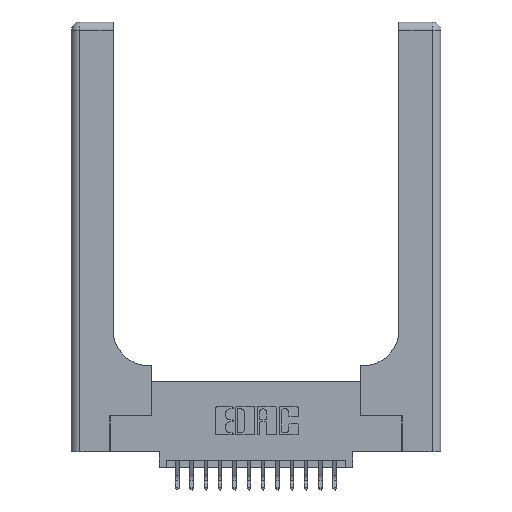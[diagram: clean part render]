
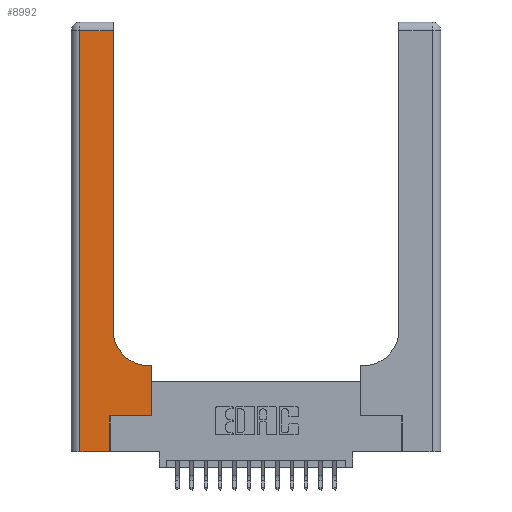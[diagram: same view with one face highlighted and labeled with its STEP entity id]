
A CAD part, top view. The second image highlights one B-rep face of the part: STEP entity #8992.
In plain terms, the highlighted planar face has unit normal (0, 0, 1).
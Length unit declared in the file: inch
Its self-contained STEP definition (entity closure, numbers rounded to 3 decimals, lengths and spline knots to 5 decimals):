
#771 = ORIENTED_EDGE ( 'NONE', *, *, #18063, .T. ) ;
#1486 = VECTOR ( 'NONE', #8762, 39.37008 ) ;
#1741 = CARTESIAN_POINT ( 'NONE',  ( 0.2915, 2.94, 0.37 ) ) ;
#1759 = VERTEX_POINT ( 'NONE', #3082 ) ;
#1882 = EDGE_CURVE ( 'NONE', #12245, #2724, #18890, .T. ) ;
#1940 = DIRECTION ( 'NONE',  ( 0., 1., 0. ) ) ;
#2143 = CARTESIAN_POINT ( 'NONE',  ( 0.269, 0., 0.37 ) ) ;
#2274 = VECTOR ( 'NONE', #14615, 39.37008 ) ;
#2296 = CARTESIAN_POINT ( 'NONE',  ( 0.5415, 0.6, 0.37 ) ) ;
#2349 = CARTESIAN_POINT ( 'NONE',  ( 0., 2.94, 0.37 ) ) ;
#2434 = ORIENTED_EDGE ( 'NONE', *, *, #6491, .T. ) ;
#2440 = VERTEX_POINT ( 'NONE', #1741 ) ;
#2676 = LINE ( 'NONE', #6686, #13928 ) ;
#2724 = VERTEX_POINT ( 'NONE', #4999 ) ;
#3082 = CARTESIAN_POINT ( 'NONE',  ( 0.5585, 0.25, 0.37 ) ) ;
#3432 = CARTESIAN_POINT ( 'NONE',  ( 0.269, 0.25, 0.37 ) ) ;
#3605 = ORIENTED_EDGE ( 'NONE', *, *, #11984, .T. ) ;
#3850 = LINE ( 'NONE', #18916, #2274 ) ;
#4032 = DIRECTION ( 'NONE',  ( 0., -1., 0. ) ) ;
#4252 = LINE ( 'NONE', #7621, #5389 ) ;
#4438 = VECTOR ( 'NONE', #16854, 39.37008 ) ;
#4523 = VERTEX_POINT ( 'NONE', #18541 ) ;
#4768 = ORIENTED_EDGE ( 'NONE', *, *, #18151, .T. ) ;
#4783 = VERTEX_POINT ( 'NONE', #13072 ) ;
#4784 = CARTESIAN_POINT ( 'NONE',  ( 0., 0., 0.37 ) ) ;
#4999 = CARTESIAN_POINT ( 'NONE',  ( 0.2915, 0.85, 0.37 ) ) ;
#5149 = VECTOR ( 'NONE', #12621, 39.37008 ) ;
#5171 = DIRECTION ( 'NONE',  ( -1., 0., 0. ) ) ;
#5389 = VECTOR ( 'NONE', #1940, 39.37008 ) ;
#5469 = ORIENTED_EDGE ( 'NONE', *, *, #11515, .T. ) ;
#5716 = EDGE_LOOP ( 'NONE', ( #2434, #6113, #771, #4768, #14386, #7467, #5469, #3605, #16945 ) ) ;
#6108 = CARTESIAN_POINT ( 'NONE',  ( 0.5585, 0.6, 0.37 ) ) ;
#6113 = ORIENTED_EDGE ( 'NONE', *, *, #17376, .T. ) ;
#6252 = VECTOR ( 'NONE', #13471, 39.37008 ) ;
#6491 = EDGE_CURVE ( 'NONE', #2724, #2440, #2676, .T. ) ;
#6592 = DIRECTION ( 'NONE',  ( 0., 0., -1. ) ) ;
#6686 = CARTESIAN_POINT ( 'NONE',  ( 0.2915, 3., 0.37 ) ) ;
#7422 = VECTOR ( 'NONE', #4032, 39.37008 ) ;
#7467 = ORIENTED_EDGE ( 'NONE', *, *, #16045, .T. ) ;
#7542 = VERTEX_POINT ( 'NONE', #3432 ) ;
#7621 = CARTESIAN_POINT ( 'NONE',  ( 0.5585, 0.25, 0.37 ) ) ;
#8762 = DIRECTION ( 'NONE',  ( -1., 0., 0. ) ) ;
#8992 = ADVANCED_FACE ( 'NONE', ( #16774 ), #12538, .F. ) ;
#9078 = LINE ( 'NONE', #2349, #5149 ) ;
#9224 = CARTESIAN_POINT ( 'NONE',  ( 0.06, 2.94, 0.37 ) ) ;
#9923 = CARTESIAN_POINT ( 'NONE',  ( 0.06, 3., 0.37 ) ) ;
#10293 = CARTESIAN_POINT ( 'NONE',  ( 0.2915, 0.6, 0.37 ) ) ;
#11515 = EDGE_CURVE ( 'NONE', #1759, #11994, #4252, .T. ) ;
#11984 = EDGE_CURVE ( 'NONE', #11994, #12245, #13197, .T. ) ;
#11994 = VERTEX_POINT ( 'NONE', #6108 ) ;
#12245 = VERTEX_POINT ( 'NONE', #2296 ) ;
#12308 = CARTESIAN_POINT ( 'NONE',  ( 0.5415, 0.85, 0.37 ) ) ;
#12538 = PLANE ( 'NONE',  #17915 ) ;
#12621 = DIRECTION ( 'NONE',  ( -1., 0., 0. ) ) ;
#12978 = LINE ( 'NONE', #2143, #4438 ) ;
#13072 = CARTESIAN_POINT ( 'NONE',  ( 0.269, 0., 0.37 ) ) ;
#13197 = LINE ( 'NONE', #10293, #1486 ) ;
#13234 = VERTEX_POINT ( 'NONE', #9224 ) ;
#13471 = DIRECTION ( 'NONE',  ( 1., 0., 0. ) ) ;
#13798 = DIRECTION ( 'NONE',  ( 0., 0., -1. ) ) ;
#13928 = VECTOR ( 'NONE', #18486, 39.37008 ) ;
#14386 = ORIENTED_EDGE ( 'NONE', *, *, #17837, .T. ) ;
#14596 = LINE ( 'NONE', #4784, #6252 ) ;
#14615 = DIRECTION ( 'NONE',  ( 1., 0., 0. ) ) ;
#16045 = EDGE_CURVE ( 'NONE', #7542, #1759, #3850, .T. ) ;
#16774 = FACE_OUTER_BOUND ( 'NONE', #5716, .T. ) ;
#16778 = DIRECTION ( 'NONE',  ( 1., 0., 0. ) ) ;
#16854 = DIRECTION ( 'NONE',  ( 0., 1., 0. ) ) ;
#16920 = CARTESIAN_POINT ( 'NONE',  ( 0., 3., 0.37 ) ) ;
#16945 = ORIENTED_EDGE ( 'NONE', *, *, #1882, .T. ) ;
#17376 = EDGE_CURVE ( 'NONE', #2440, #13234, #9078, .T. ) ;
#17837 = EDGE_CURVE ( 'NONE', #4783, #7542, #12978, .T. ) ;
#17915 = AXIS2_PLACEMENT_3D ( 'NONE', #16920, #6592, #5171 ) ;
#18063 = EDGE_CURVE ( 'NONE', #13234, #4523, #18727, .T. ) ;
#18151 = EDGE_CURVE ( 'NONE', #4523, #4783, #14596, .T. ) ;
#18486 = DIRECTION ( 'NONE',  ( 0., 1., 0. ) ) ;
#18541 = CARTESIAN_POINT ( 'NONE',  ( 0.06, 0., 0.37 ) ) ;
#18727 = LINE ( 'NONE', #9923, #7422 ) ;
#18890 = CIRCLE ( 'NONE', #18943, 0.25 ) ;
#18916 = CARTESIAN_POINT ( 'NONE',  ( 0.269, 0.25, 0.37 ) ) ;
#18943 = AXIS2_PLACEMENT_3D ( 'NONE', #12308, #13798, #16778 ) ;
